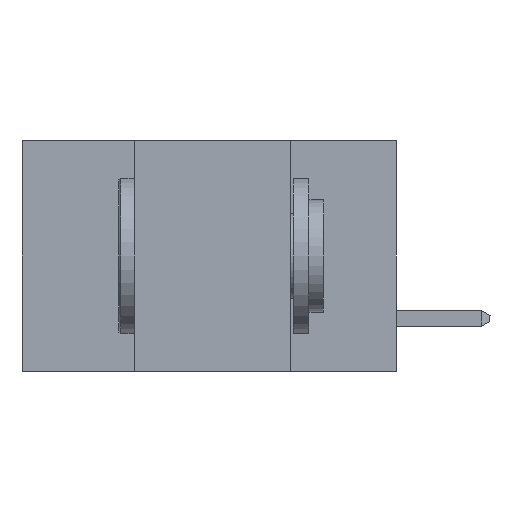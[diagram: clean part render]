
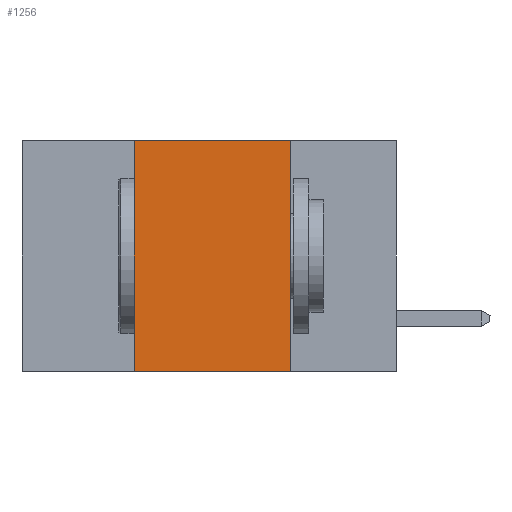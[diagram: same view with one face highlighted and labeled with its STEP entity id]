
A CAD part, left-side view. The second image highlights one B-rep face of the part: STEP entity #1256.
In plain terms, the highlighted planar face has unit normal (-1, 0, 0).
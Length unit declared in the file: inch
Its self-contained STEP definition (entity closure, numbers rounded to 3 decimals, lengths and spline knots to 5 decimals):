
#211 = EDGE_LOOP ( 'NONE', ( #9474, #289, #10129, #14304 ) ) ;
#289 = ORIENTED_EDGE ( 'NONE', *, *, #5711, .F. ) ;
#769 = DIRECTION ( 'NONE',  ( 1., 0., 0. ) ) ;
#964 = EDGE_CURVE ( 'NONE', #4074, #1425, #6876, .T. ) ;
#1256 = ADVANCED_FACE ( 'NONE', ( #16101 ), #13817, .F. ) ;
#1425 = VERTEX_POINT ( 'NONE', #14374 ) ;
#2217 = DIRECTION ( 'NONE',  ( 0., 0., -1. ) ) ;
#2291 = AXIS2_PLACEMENT_3D ( 'NONE', #2573, #769, #15073 ) ;
#2573 = CARTESIAN_POINT ( 'NONE',  ( 0., 0.6, 0. ) ) ;
#3025 = VECTOR ( 'NONE', #2217, 39.37008 ) ;
#3080 = VERTEX_POINT ( 'NONE', #9737 ) ;
#3529 = VECTOR ( 'NONE', #11289, 39.37008 ) ;
#4074 = VERTEX_POINT ( 'NONE', #5079 ) ;
#5079 = CARTESIAN_POINT ( 'NONE',  ( 0., 0.17, 0. ) ) ;
#5687 = VECTOR ( 'NONE', #11785, 39.37008 ) ;
#5711 = EDGE_CURVE ( 'NONE', #3080, #4074, #7838, .T. ) ;
#6081 = CARTESIAN_POINT ( 'NONE',  ( 0., 0.42, -0.37 ) ) ;
#6876 = LINE ( 'NONE', #11293, #3025 ) ;
#7838 = LINE ( 'NONE', #11252, #3529 ) ;
#8221 = CARTESIAN_POINT ( 'NONE',  ( 0., 0.42, -0.37 ) ) ;
#8289 = EDGE_CURVE ( 'NONE', #17388, #1425, #16934, .T. ) ;
#9474 = ORIENTED_EDGE ( 'NONE', *, *, #964, .F. ) ;
#9586 = EDGE_CURVE ( 'NONE', #17388, #3080, #17532, .T. ) ;
#9737 = CARTESIAN_POINT ( 'NONE',  ( 0., 0.42, 0. ) ) ;
#10129 = ORIENTED_EDGE ( 'NONE', *, *, #9586, .F. ) ;
#11252 = CARTESIAN_POINT ( 'NONE',  ( 0., 0.6, 0. ) ) ;
#11289 = DIRECTION ( 'NONE',  ( 0., -1., 0. ) ) ;
#11293 = CARTESIAN_POINT ( 'NONE',  ( 0., 0.17, -0.37 ) ) ;
#11785 = DIRECTION ( 'NONE',  ( 0., -1., 0. ) ) ;
#11828 = CARTESIAN_POINT ( 'NONE',  ( 0., 0.6, -0.37 ) ) ;
#13817 = PLANE ( 'NONE',  #2291 ) ;
#13870 = VECTOR ( 'NONE', #16586, 39.37008 ) ;
#14304 = ORIENTED_EDGE ( 'NONE', *, *, #8289, .T. ) ;
#14374 = CARTESIAN_POINT ( 'NONE',  ( 0., 0.17, -0.37 ) ) ;
#15073 = DIRECTION ( 'NONE',  ( 0., 0., -1. ) ) ;
#16101 = FACE_OUTER_BOUND ( 'NONE', #211, .T. ) ;
#16586 = DIRECTION ( 'NONE',  ( 0., 0., 1. ) ) ;
#16934 = LINE ( 'NONE', #11828, #5687 ) ;
#17388 = VERTEX_POINT ( 'NONE', #6081 ) ;
#17532 = LINE ( 'NONE', #8221, #13870 ) ;
